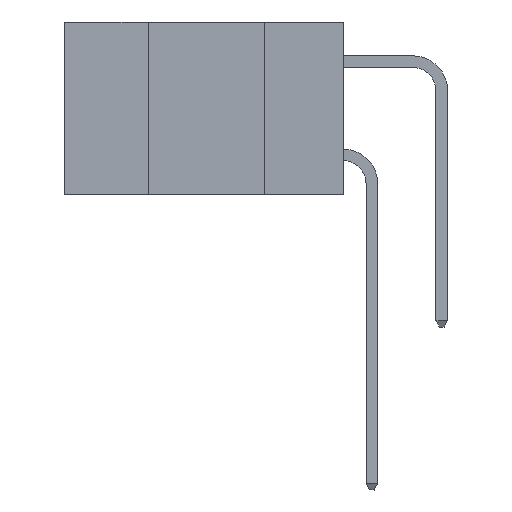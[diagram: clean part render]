
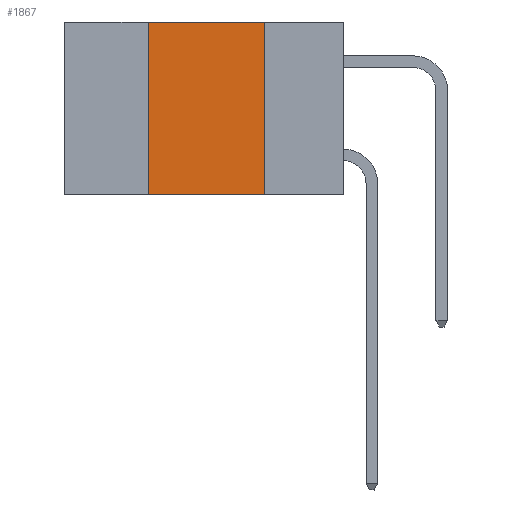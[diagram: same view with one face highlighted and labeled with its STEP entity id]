
A CAD part, left-side view. The second image highlights one B-rep face of the part: STEP entity #1867.
In plain terms, the highlighted planar face has unit normal (-1, 0, 0).
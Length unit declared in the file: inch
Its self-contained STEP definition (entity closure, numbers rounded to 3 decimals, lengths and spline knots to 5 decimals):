
#368 = EDGE_LOOP ( 'NONE', ( #15961, #17345, #8544, #9181 ) ) ;
#446 = VECTOR ( 'NONE', #5734, 39.37008 ) ;
#973 = CARTESIAN_POINT ( 'NONE',  ( 0., 0.6, -0.37 ) ) ;
#1180 = VECTOR ( 'NONE', #11633, 39.37008 ) ;
#1592 = VERTEX_POINT ( 'NONE', #6976 ) ;
#1782 = DIRECTION ( 'NONE',  ( 1., 0., 0. ) ) ;
#1867 = ADVANCED_FACE ( 'NONE', ( #6266 ), #6283, .F. ) ;
#2245 = CARTESIAN_POINT ( 'NONE',  ( 0., 0.17, 0. ) ) ;
#2963 = CARTESIAN_POINT ( 'NONE',  ( 0., 0.17, -0.37 ) ) ;
#3005 = EDGE_CURVE ( 'NONE', #8658, #4793, #12189, .T. ) ;
#4422 = CARTESIAN_POINT ( 'NONE',  ( 0., 0.6, 0. ) ) ;
#4793 = VERTEX_POINT ( 'NONE', #2963 ) ;
#4913 = EDGE_CURVE ( 'NONE', #9268, #8658, #8709, .T. ) ;
#5410 = CARTESIAN_POINT ( 'NONE',  ( 0., 0.17, 0. ) ) ;
#5734 = DIRECTION ( 'NONE',  ( 0., 0., 1. ) ) ;
#5901 = LINE ( 'NONE', #18865, #446 ) ;
#6073 = EDGE_CURVE ( 'NONE', #1592, #9268, #5901, .T. ) ;
#6266 = FACE_OUTER_BOUND ( 'NONE', #368, .T. ) ;
#6283 = PLANE ( 'NONE',  #15570 ) ;
#6976 = CARTESIAN_POINT ( 'NONE',  ( 0., 0.42, -0.37 ) ) ;
#8038 = VECTOR ( 'NONE', #16917, 39.37008 ) ;
#8148 = CARTESIAN_POINT ( 'NONE',  ( 0., 0.42, 0. ) ) ;
#8544 = ORIENTED_EDGE ( 'NONE', *, *, #6073, .F. ) ;
#8658 = VERTEX_POINT ( 'NONE', #2245 ) ;
#8709 = LINE ( 'NONE', #4422, #1180 ) ;
#9181 = ORIENTED_EDGE ( 'NONE', *, *, #12457, .T. ) ;
#9209 = LINE ( 'NONE', #973, #8038 ) ;
#9268 = VERTEX_POINT ( 'NONE', #8148 ) ;
#11633 = DIRECTION ( 'NONE',  ( 0., -1., 0. ) ) ;
#12189 = LINE ( 'NONE', #5410, #15411 ) ;
#12193 = CARTESIAN_POINT ( 'NONE',  ( 0., 0.6, 0. ) ) ;
#12457 = EDGE_CURVE ( 'NONE', #1592, #4793, #9209, .T. ) ;
#13601 = DIRECTION ( 'NONE',  ( 0., 0., -1. ) ) ;
#15411 = VECTOR ( 'NONE', #18529, 39.37008 ) ;
#15570 = AXIS2_PLACEMENT_3D ( 'NONE', #12193, #1782, #13601 ) ;
#15961 = ORIENTED_EDGE ( 'NONE', *, *, #3005, .F. ) ;
#16917 = DIRECTION ( 'NONE',  ( 0., -1., 0. ) ) ;
#17345 = ORIENTED_EDGE ( 'NONE', *, *, #4913, .F. ) ;
#18529 = DIRECTION ( 'NONE',  ( 0., 0., -1. ) ) ;
#18865 = CARTESIAN_POINT ( 'NONE',  ( 0., 0.42, 0. ) ) ;
